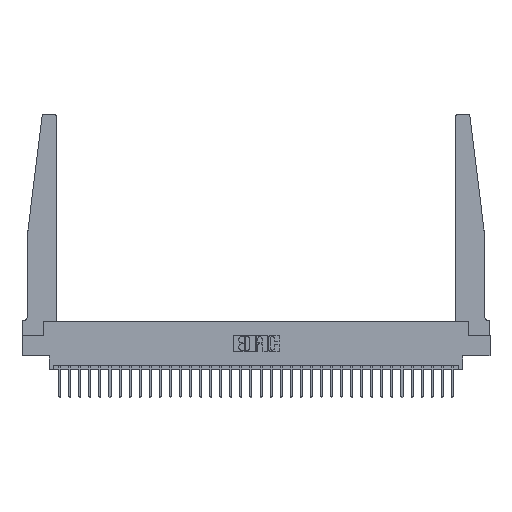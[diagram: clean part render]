
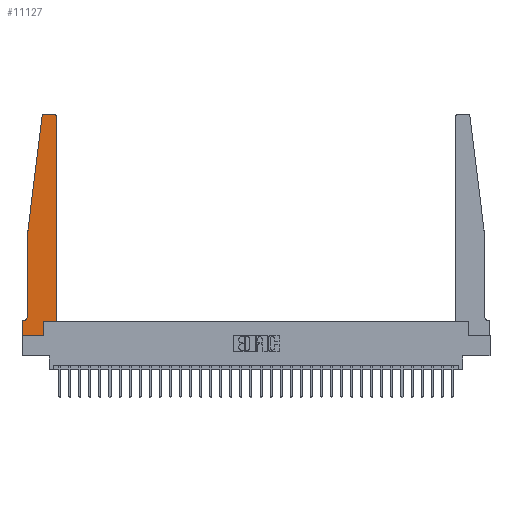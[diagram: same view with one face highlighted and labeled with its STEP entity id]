
A CAD part, top view. The second image highlights one B-rep face of the part: STEP entity #11127.
In plain terms, the highlighted planar face has unit normal (0, 0, 1).
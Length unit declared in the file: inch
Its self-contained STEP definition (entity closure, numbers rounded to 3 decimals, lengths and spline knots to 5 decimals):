
#372 = VERTEX_POINT ( 'NONE', #4980 ) ;
#504 = DIRECTION ( 'NONE',  ( -1., 0., 0. ) ) ;
#954 = DIRECTION ( 'NONE',  ( 0., 1., 0. ) ) ;
#1135 = EDGE_CURVE ( 'NONE', #30097, #6470, #3545, .T. ) ;
#1137 = EDGE_CURVE ( 'NONE', #16991, #28529, #28435, .T. ) ;
#1169 = CARTESIAN_POINT ( 'NONE',  ( 0.395, 2.75, 0.37 ) ) ;
#1894 = CARTESIAN_POINT ( 'NONE',  ( 0.015, 0.2375, 0.37 ) ) ;
#2570 = EDGE_CURVE ( 'NONE', #30121, #372, #15615, .T. ) ;
#2700 = LINE ( 'NONE', #7844, #20541 ) ;
#2765 = VECTOR ( 'NONE', #10171, 39.37008 ) ;
#2907 = LINE ( 'NONE', #8181, #21462 ) ;
#2982 = EDGE_CURVE ( 'NONE', #372, #30097, #19331, .T. ) ;
#3349 = VERTEX_POINT ( 'NONE', #25686 ) ;
#3378 = EDGE_CURVE ( 'NONE', #25552, #18908, #27184, .T. ) ;
#3545 = LINE ( 'NONE', #17350, #2765 ) ;
#3693 = AXIS2_PLACEMENT_3D ( 'NONE', #8776, #25607, #11224 ) ;
#4357 = DIRECTION ( 'NONE',  ( -1., 0., 0. ) ) ;
#4500 = LINE ( 'NONE', #27457, #11021 ) ;
#4980 = CARTESIAN_POINT ( 'NONE',  ( 0., 0., 0.37 ) ) ;
#5332 = CARTESIAN_POINT ( 'NONE',  ( 0., 0.1875, 0.37 ) ) ;
#5355 = ORIENTED_EDGE ( 'NONE', *, *, #12985, .T. ) ;
#5494 = DIRECTION ( 'NONE',  ( -0.122, -0.992, 0. ) ) ;
#5589 = ORIENTED_EDGE ( 'NONE', *, *, #22424, .T. ) ;
#6470 = VERTEX_POINT ( 'NONE', #13948 ) ;
#6477 = VECTOR ( 'NONE', #15466, 39.37008 ) ;
#7245 = VERTEX_POINT ( 'NONE', #14632 ) ;
#7844 = CARTESIAN_POINT ( 'NONE',  ( 0.065, 1.25, 0.37 ) ) ;
#8181 = CARTESIAN_POINT ( 'NONE',  ( 0.425, 0.18, 0.37 ) ) ;
#8290 = ORIENTED_EDGE ( 'NONE', *, *, #13676, .T. ) ;
#8522 = EDGE_CURVE ( 'NONE', #28529, #27977, #25387, .T. ) ;
#8776 = CARTESIAN_POINT ( 'NONE',  ( 0.395, 2.72, 0.37 ) ) ;
#8788 = CIRCLE ( 'NONE', #3693, 0.03 ) ;
#9930 = ORIENTED_EDGE ( 'NONE', *, *, #8522, .T. ) ;
#10091 = CIRCLE ( 'NONE', #10820, 0.03 ) ;
#10123 = DIRECTION ( 'NONE',  ( 0., 0., 1. ) ) ;
#10171 = DIRECTION ( 'NONE',  ( 0., 1., 0. ) ) ;
#10338 = DIRECTION ( 'NONE',  ( 1., 0., 0. ) ) ;
#10641 = DIRECTION ( 'NONE',  ( 1., 0., 0. ) ) ;
#10820 = AXIS2_PLACEMENT_3D ( 'NONE', #24520, #10123, #26939 ) ;
#11021 = VECTOR ( 'NONE', #954, 39.37008 ) ;
#11127 = ADVANCED_FACE ( 'NONE', ( #25519 ), #22335, .T. ) ;
#11186 = AXIS2_PLACEMENT_3D ( 'NONE', #1894, #18878, #4357 ) ;
#11224 = DIRECTION ( 'NONE',  ( 1., 0., 0. ) ) ;
#12673 = CARTESIAN_POINT ( 'NONE',  ( 0.065, 0.1875, 0.37 ) ) ;
#12985 = EDGE_CURVE ( 'NONE', #27531, #16991, #2700, .T. ) ;
#13044 = CARTESIAN_POINT ( 'NONE',  ( 0., 0., 0.37 ) ) ;
#13097 = EDGE_LOOP ( 'NONE', ( #20481, #5589, #5355, #15769, #9930, #28535, #13652, #26908, #19125, #28211, #18110, #8290 ) ) ;
#13635 = CARTESIAN_POINT ( 'NONE',  ( 0.015, 0.1875, 0.37 ) ) ;
#13652 = ORIENTED_EDGE ( 'NONE', *, *, #2570, .T. ) ;
#13676 = EDGE_CURVE ( 'NONE', #7245, #25552, #8788, .T. ) ;
#13948 = CARTESIAN_POINT ( 'NONE',  ( 0.2605, 0.18, 0.37 ) ) ;
#14632 = CARTESIAN_POINT ( 'NONE',  ( 0.425, 2.72, 0.37 ) ) ;
#15037 = DIRECTION ( 'NONE',  ( 0., -1., 0. ) ) ;
#15466 = DIRECTION ( 'NONE',  ( 1., 0., 0. ) ) ;
#15600 = CARTESIAN_POINT ( 'NONE',  ( 0.065, 0.2375, 0.37 ) ) ;
#15615 = LINE ( 'NONE', #18440, #27602 ) ;
#15769 = ORIENTED_EDGE ( 'NONE', *, *, #1137, .T. ) ;
#16012 = DIRECTION ( 'NONE',  ( 0., -1., 0. ) ) ;
#16991 = VERTEX_POINT ( 'NONE', #29084 ) ;
#17350 = CARTESIAN_POINT ( 'NONE',  ( 0.2605, 0.18, 0.37 ) ) ;
#17515 = CARTESIAN_POINT ( 'NONE',  ( 0., 0.1875, 0.37 ) ) ;
#18110 = ORIENTED_EDGE ( 'NONE', *, *, #20031, .T. ) ;
#18440 = CARTESIAN_POINT ( 'NONE',  ( 0., 0., 0.37 ) ) ;
#18872 = CARTESIAN_POINT ( 'NONE',  ( 0.25, 2.75, 0.37 ) ) ;
#18878 = DIRECTION ( 'NONE',  ( 0., 0., -1. ) ) ;
#18908 = VERTEX_POINT ( 'NONE', #30882 ) ;
#19125 = ORIENTED_EDGE ( 'NONE', *, *, #1135, .T. ) ;
#19331 = LINE ( 'NONE', #13044, #6477 ) ;
#19673 = VECTOR ( 'NONE', #504, 39.37008 ) ;
#19938 = EDGE_CURVE ( 'NONE', #27977, #30121, #26787, .T. ) ;
#20031 = EDGE_CURVE ( 'NONE', #3349, #7245, #4500, .T. ) ;
#20481 = ORIENTED_EDGE ( 'NONE', *, *, #3378, .T. ) ;
#20541 = VECTOR ( 'NONE', #5494, 39.37008 ) ;
#20829 = VECTOR ( 'NONE', #30817, 39.37008 ) ;
#21322 = VECTOR ( 'NONE', #15037, 39.37008 ) ;
#21462 = VECTOR ( 'NONE', #10641, 39.37008 ) ;
#22150 = CARTESIAN_POINT ( 'NONE',  ( 0.2605, 0., 0.37 ) ) ;
#22335 = PLANE ( 'NONE',  #27897 ) ;
#22424 = EDGE_CURVE ( 'NONE', #18908, #27531, #10091, .T. ) ;
#24021 = CARTESIAN_POINT ( 'NONE',  ( 0.24675, 2.72367, 0.37 ) ) ;
#24520 = CARTESIAN_POINT ( 'NONE',  ( 0.27653, 2.72, 0.37 ) ) ;
#24729 = DIRECTION ( 'NONE',  ( 0., 0., 1. ) ) ;
#25387 = CIRCLE ( 'NONE', #11186, 0.05 ) ;
#25519 = FACE_OUTER_BOUND ( 'NONE', #13097, .T. ) ;
#25552 = VERTEX_POINT ( 'NONE', #1169 ) ;
#25607 = DIRECTION ( 'NONE',  ( 0., 0., 1. ) ) ;
#25686 = CARTESIAN_POINT ( 'NONE',  ( 0.425, 0.18, 0.37 ) ) ;
#26084 = EDGE_CURVE ( 'NONE', #6470, #3349, #2907, .T. ) ;
#26787 = LINE ( 'NONE', #12673, #19673 ) ;
#26908 = ORIENTED_EDGE ( 'NONE', *, *, #2982, .T. ) ;
#26939 = DIRECTION ( 'NONE',  ( 1., 0., 0. ) ) ;
#26988 = CARTESIAN_POINT ( 'NONE',  ( 0.065, 1.25, 0.37 ) ) ;
#27184 = LINE ( 'NONE', #18872, #20829 ) ;
#27457 = CARTESIAN_POINT ( 'NONE',  ( 0.425, 0.18, 0.37 ) ) ;
#27531 = VERTEX_POINT ( 'NONE', #24021 ) ;
#27602 = VECTOR ( 'NONE', #16012, 39.37008 ) ;
#27897 = AXIS2_PLACEMENT_3D ( 'NONE', #17515, #24729, #10338 ) ;
#27977 = VERTEX_POINT ( 'NONE', #13635 ) ;
#28211 = ORIENTED_EDGE ( 'NONE', *, *, #26084, .T. ) ;
#28435 = LINE ( 'NONE', #26988, #21322 ) ;
#28529 = VERTEX_POINT ( 'NONE', #15600 ) ;
#28535 = ORIENTED_EDGE ( 'NONE', *, *, #19938, .T. ) ;
#29084 = CARTESIAN_POINT ( 'NONE',  ( 0.065, 1.25, 0.37 ) ) ;
#30097 = VERTEX_POINT ( 'NONE', #22150 ) ;
#30121 = VERTEX_POINT ( 'NONE', #5332 ) ;
#30817 = DIRECTION ( 'NONE',  ( -1., 0., 0. ) ) ;
#30882 = CARTESIAN_POINT ( 'NONE',  ( 0.27653, 2.75, 0.37 ) ) ;
